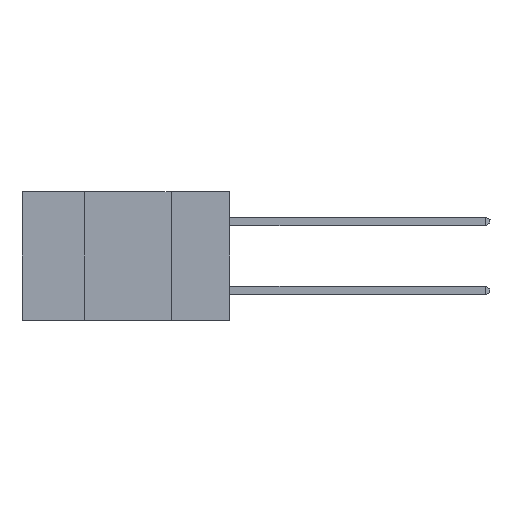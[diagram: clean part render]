
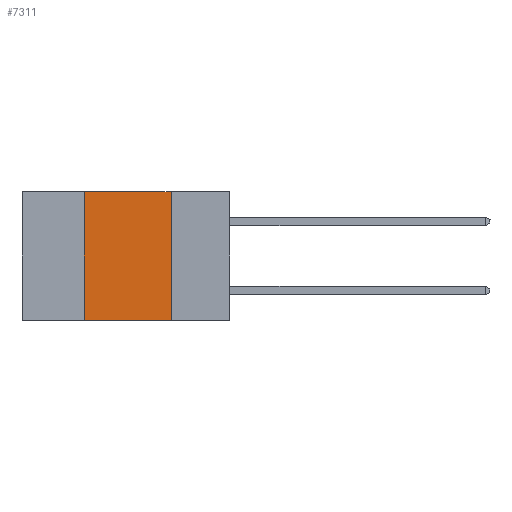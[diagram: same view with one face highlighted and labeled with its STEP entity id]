
A CAD part, left-side view. The second image highlights one B-rep face of the part: STEP entity #7311.
In plain terms, the highlighted planar face has unit normal (-1, 0, 0).
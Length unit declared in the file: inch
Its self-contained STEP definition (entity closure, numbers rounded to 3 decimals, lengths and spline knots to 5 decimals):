
#501 = CARTESIAN_POINT ( 'NONE',  ( 0., 0.42, -0.37 ) ) ;
#633 = VECTOR ( 'NONE', #11124, 39.37008 ) ;
#734 = CARTESIAN_POINT ( 'NONE',  ( 0., 0.6, -0.37 ) ) ;
#1373 = VECTOR ( 'NONE', #3890, 39.37008 ) ;
#1752 = DIRECTION ( 'NONE',  ( 0., -1., 0. ) ) ;
#2129 = EDGE_CURVE ( 'NONE', #4634, #2919, #2662, .T. ) ;
#2546 = VECTOR ( 'NONE', #6971, 39.37008 ) ;
#2662 = LINE ( 'NONE', #2859, #2546 ) ;
#2773 = EDGE_CURVE ( 'NONE', #4133, #4634, #5077, .T. ) ;
#2859 = CARTESIAN_POINT ( 'NONE',  ( 0., 0.6, 0. ) ) ;
#2919 = VERTEX_POINT ( 'NONE', #6278 ) ;
#3317 = EDGE_CURVE ( 'NONE', #4133, #11565, #6813, .T. ) ;
#3655 = CARTESIAN_POINT ( 'NONE',  ( 0., 0.6, 0. ) ) ;
#3682 = ORIENTED_EDGE ( 'NONE', *, *, #2129, .F. ) ;
#3864 = EDGE_CURVE ( 'NONE', #2919, #11565, #4983, .T. ) ;
#3890 = DIRECTION ( 'NONE',  ( 0., 0., -1. ) ) ;
#4133 = VERTEX_POINT ( 'NONE', #501 ) ;
#4634 = VERTEX_POINT ( 'NONE', #6890 ) ;
#4983 = LINE ( 'NONE', #8076, #1373 ) ;
#5077 = LINE ( 'NONE', #6090, #633 ) ;
#5671 = VECTOR ( 'NONE', #1752, 39.37008 ) ;
#6090 = CARTESIAN_POINT ( 'NONE',  ( 0., 0.42, -0.37 ) ) ;
#6278 = CARTESIAN_POINT ( 'NONE',  ( 0., 0.17, 0. ) ) ;
#6577 = AXIS2_PLACEMENT_3D ( 'NONE', #3655, #12720, #10676 ) ;
#6813 = LINE ( 'NONE', #734, #5671 ) ;
#6890 = CARTESIAN_POINT ( 'NONE',  ( 0., 0.42, 0. ) ) ;
#6971 = DIRECTION ( 'NONE',  ( 0., -1., 0. ) ) ;
#7311 = ADVANCED_FACE ( 'NONE', ( #8717 ), #9743, .F. ) ;
#7580 = ORIENTED_EDGE ( 'NONE', *, *, #3317, .T. ) ;
#8076 = CARTESIAN_POINT ( 'NONE',  ( 0., 0.17, -0.37 ) ) ;
#8717 = FACE_OUTER_BOUND ( 'NONE', #11006, .T. ) ;
#8878 = ORIENTED_EDGE ( 'NONE', *, *, #3864, .F. ) ;
#9743 = PLANE ( 'NONE',  #6577 ) ;
#10676 = DIRECTION ( 'NONE',  ( 0., 0., -1. ) ) ;
#11006 = EDGE_LOOP ( 'NONE', ( #8878, #3682, #12988, #7580 ) ) ;
#11124 = DIRECTION ( 'NONE',  ( 0., 0., 1. ) ) ;
#11565 = VERTEX_POINT ( 'NONE', #13041 ) ;
#12720 = DIRECTION ( 'NONE',  ( 1., 0., 0. ) ) ;
#12988 = ORIENTED_EDGE ( 'NONE', *, *, #2773, .F. ) ;
#13041 = CARTESIAN_POINT ( 'NONE',  ( 0., 0.17, -0.37 ) ) ;
